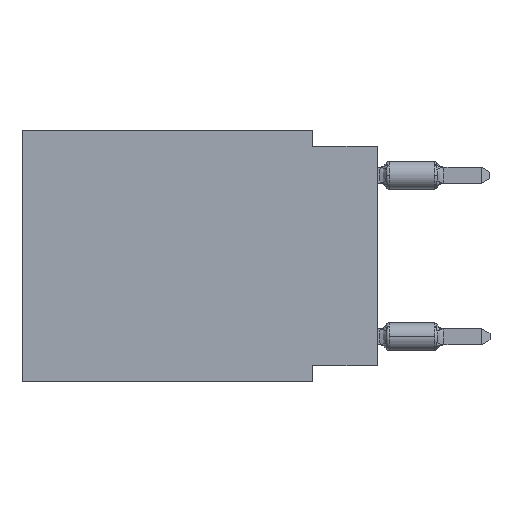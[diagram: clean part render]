
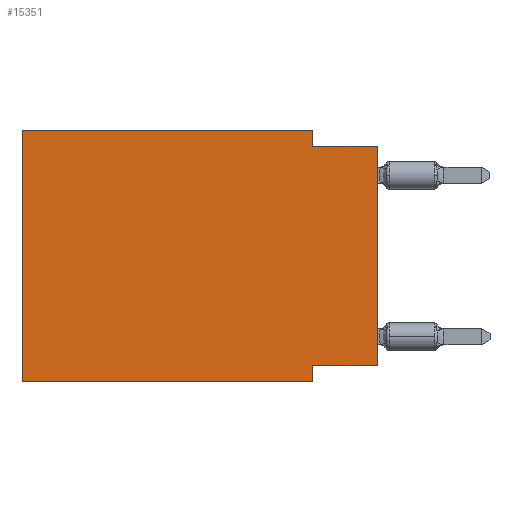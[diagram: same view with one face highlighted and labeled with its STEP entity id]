
A CAD part, left-side view. The second image highlights one B-rep face of the part: STEP entity #15351.
In plain terms, the highlighted planar face has unit normal (-1, 0, 0).
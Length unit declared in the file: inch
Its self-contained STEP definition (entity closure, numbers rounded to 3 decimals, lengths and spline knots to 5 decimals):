
#66 = ORIENTED_EDGE ( 'NONE', *, *, #16731, .F. ) ;
#289 = VERTEX_POINT ( 'NONE', #12679 ) ;
#334 = CARTESIAN_POINT ( 'NONE',  ( 0., 0.1, -0.39 ) ) ;
#1089 = CARTESIAN_POINT ( 'NONE',  ( 0., 0.1, -0.365 ) ) ;
#1115 = VECTOR ( 'NONE', #10264, 39.37008 ) ;
#2751 = EDGE_CURVE ( 'NONE', #12012, #10992, #11653, .T. ) ;
#2773 = CARTESIAN_POINT ( 'NONE',  ( 0., 0.55, 0. ) ) ;
#3128 = LINE ( 'NONE', #334, #13115 ) ;
#3310 = CARTESIAN_POINT ( 'NONE',  ( 0., 0.55, 0. ) ) ;
#3610 = EDGE_CURVE ( 'NONE', #10992, #9233, #13225, .T. ) ;
#3654 = AXIS2_PLACEMENT_3D ( 'NONE', #3310, #15977, #10344 ) ;
#3725 = EDGE_LOOP ( 'NONE', ( #9855, #9240, #14173, #66, #10195, #4198, #15060, #16297 ) ) ;
#3747 = VECTOR ( 'NONE', #6357, 39.37008 ) ;
#4099 = CARTESIAN_POINT ( 'NONE',  ( 0., 0., -0.025 ) ) ;
#4198 = ORIENTED_EDGE ( 'NONE', *, *, #16898, .T. ) ;
#4218 = VECTOR ( 'NONE', #8069, 39.37008 ) ;
#4961 = LINE ( 'NONE', #14278, #1115 ) ;
#5143 = VERTEX_POINT ( 'NONE', #12709 ) ;
#5197 = CARTESIAN_POINT ( 'NONE',  ( 0., 0.1, 0. ) ) ;
#5371 = LINE ( 'NONE', #2773, #4218 ) ;
#5408 = CARTESIAN_POINT ( 'NONE',  ( 0., 0.55, 0. ) ) ;
#6357 = DIRECTION ( 'NONE',  ( 0., -1., 0. ) ) ;
#6442 = VERTEX_POINT ( 'NONE', #9582 ) ;
#6718 = LINE ( 'NONE', #5408, #10559 ) ;
#6732 = VECTOR ( 'NONE', #11282, 39.37008 ) ;
#7467 = DIRECTION ( 'NONE',  ( 0., 0., -1. ) ) ;
#8069 = DIRECTION ( 'NONE',  ( 0., -1., 0. ) ) ;
#8322 = CARTESIAN_POINT ( 'NONE',  ( 0., 0.1, -0.025 ) ) ;
#9233 = VERTEX_POINT ( 'NONE', #4099 ) ;
#9240 = ORIENTED_EDGE ( 'NONE', *, *, #3610, .F. ) ;
#9393 = VECTOR ( 'NONE', #7467, 39.37008 ) ;
#9582 = CARTESIAN_POINT ( 'NONE',  ( 0., 0.55, 0. ) ) ;
#9771 = VECTOR ( 'NONE', #10186, 39.37008 ) ;
#9855 = ORIENTED_EDGE ( 'NONE', *, *, #11986, .T. ) ;
#10186 = DIRECTION ( 'NONE',  ( 0., 1., 0. ) ) ;
#10195 = ORIENTED_EDGE ( 'NONE', *, *, #14648, .F. ) ;
#10264 = DIRECTION ( 'NONE',  ( 0., 0., 1. ) ) ;
#10344 = DIRECTION ( 'NONE',  ( 0., 0., -1. ) ) ;
#10559 = VECTOR ( 'NONE', #13514, 39.37008 ) ;
#10981 = VERTEX_POINT ( 'NONE', #16224 ) ;
#10992 = VERTEX_POINT ( 'NONE', #8322 ) ;
#11157 = VERTEX_POINT ( 'NONE', #1089 ) ;
#11282 = DIRECTION ( 'NONE',  ( 0., -1., 0. ) ) ;
#11653 = LINE ( 'NONE', #5197, #9393 ) ;
#11986 = EDGE_CURVE ( 'NONE', #10981, #9233, #4961, .T. ) ;
#12012 = VERTEX_POINT ( 'NONE', #14195 ) ;
#12679 = CARTESIAN_POINT ( 'NONE',  ( 0., 0.55, -0.39 ) ) ;
#12709 = CARTESIAN_POINT ( 'NONE',  ( 0., 0.1, -0.39 ) ) ;
#13115 = VECTOR ( 'NONE', #13560, 39.37008 ) ;
#13225 = LINE ( 'NONE', #15930, #3747 ) ;
#13514 = DIRECTION ( 'NONE',  ( 0., 0., 1. ) ) ;
#13560 = DIRECTION ( 'NONE',  ( 0., 0., -1. ) ) ;
#13902 = CARTESIAN_POINT ( 'NONE',  ( 0., 0.55, -0.39 ) ) ;
#14173 = ORIENTED_EDGE ( 'NONE', *, *, #2751, .F. ) ;
#14195 = CARTESIAN_POINT ( 'NONE',  ( 0., 0.1, 0. ) ) ;
#14249 = LINE ( 'NONE', #13902, #6732 ) ;
#14278 = CARTESIAN_POINT ( 'NONE',  ( 0., 0., 0. ) ) ;
#14648 = EDGE_CURVE ( 'NONE', #289, #6442, #6718, .T. ) ;
#15060 = ORIENTED_EDGE ( 'NONE', *, *, #16790, .F. ) ;
#15234 = FACE_OUTER_BOUND ( 'NONE', #3725, .T. ) ;
#15351 = ADVANCED_FACE ( 'NONE', ( #15234 ), #16509, .F. ) ;
#15425 = LINE ( 'NONE', #16782, #9771 ) ;
#15930 = CARTESIAN_POINT ( 'NONE',  ( 0., 0., -0.025 ) ) ;
#15977 = DIRECTION ( 'NONE',  ( 1., 0., 0. ) ) ;
#16130 = EDGE_CURVE ( 'NONE', #10981, #11157, #15425, .T. ) ;
#16224 = CARTESIAN_POINT ( 'NONE',  ( 0., 0., -0.365 ) ) ;
#16297 = ORIENTED_EDGE ( 'NONE', *, *, #16130, .F. ) ;
#16509 = PLANE ( 'NONE',  #3654 ) ;
#16731 = EDGE_CURVE ( 'NONE', #6442, #12012, #5371, .T. ) ;
#16782 = CARTESIAN_POINT ( 'NONE',  ( 0., 0., -0.365 ) ) ;
#16790 = EDGE_CURVE ( 'NONE', #11157, #5143, #3128, .T. ) ;
#16898 = EDGE_CURVE ( 'NONE', #289, #5143, #14249, .T. ) ;
